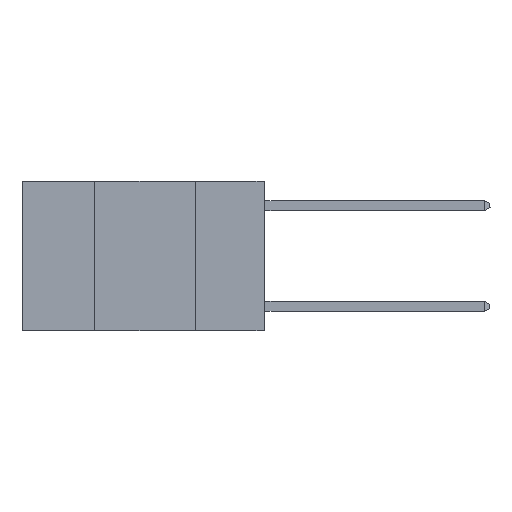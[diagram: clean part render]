
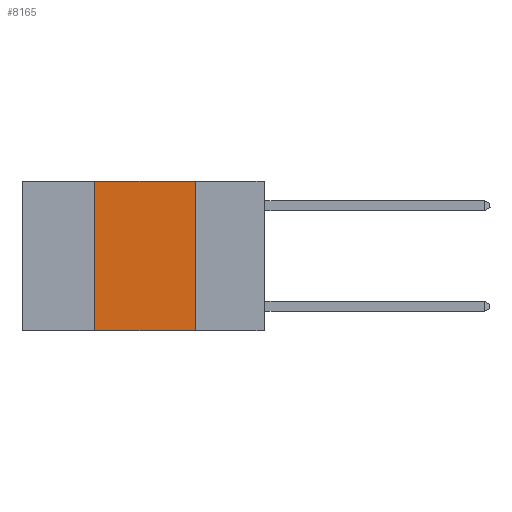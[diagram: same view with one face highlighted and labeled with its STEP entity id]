
A CAD part, left-side view. The second image highlights one B-rep face of the part: STEP entity #8165.
In plain terms, the highlighted planar face has unit normal (-1, 0, 0).
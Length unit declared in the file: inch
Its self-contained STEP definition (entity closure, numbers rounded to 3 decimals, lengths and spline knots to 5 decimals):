
#503 = VECTOR ( 'NONE', #14756, 39.37008 ) ;
#889 = EDGE_CURVE ( 'NONE', #12128, #11529, #6515, .T. ) ;
#1473 = DIRECTION ( 'NONE',  ( 1., 0., 0. ) ) ;
#2591 = LINE ( 'NONE', #10901, #12877 ) ;
#3514 = LINE ( 'NONE', #3732, #9377 ) ;
#3732 = CARTESIAN_POINT ( 'NONE',  ( 0., 0.6, -0.37 ) ) ;
#4148 = CARTESIAN_POINT ( 'NONE',  ( 0., 0.6, 0. ) ) ;
#4166 = DIRECTION ( 'NONE',  ( 0., 0., 1. ) ) ;
#4298 = CARTESIAN_POINT ( 'NONE',  ( 0., 0.17, -0.37 ) ) ;
#5715 = CARTESIAN_POINT ( 'NONE',  ( 0., 0.42, 0. ) ) ;
#6105 = VECTOR ( 'NONE', #14908, 39.37008 ) ;
#6139 = AXIS2_PLACEMENT_3D ( 'NONE', #14839, #1473, #10809 ) ;
#6515 = LINE ( 'NONE', #4148, #6105 ) ;
#6765 = PLANE ( 'NONE',  #6139 ) ;
#6842 = VERTEX_POINT ( 'NONE', #4298 ) ;
#7794 = FACE_OUTER_BOUND ( 'NONE', #10103, .T. ) ;
#8024 = CARTESIAN_POINT ( 'NONE',  ( 0., 0.17, 0. ) ) ;
#8165 = ADVANCED_FACE ( 'NONE', ( #7794 ), #6765, .F. ) ;
#8850 = EDGE_CURVE ( 'NONE', #11529, #6842, #14737, .T. ) ;
#9377 = VECTOR ( 'NONE', #14471, 39.37008 ) ;
#10103 = EDGE_LOOP ( 'NONE', ( #13173, #13599, #10405, #10841 ) ) ;
#10405 = ORIENTED_EDGE ( 'NONE', *, *, #16078, .F. ) ;
#10809 = DIRECTION ( 'NONE',  ( 0., 0., -1. ) ) ;
#10841 = ORIENTED_EDGE ( 'NONE', *, *, #11829, .T. ) ;
#10901 = CARTESIAN_POINT ( 'NONE',  ( 0., 0.42, 0. ) ) ;
#11400 = CARTESIAN_POINT ( 'NONE',  ( 0., 0.42, -0.37 ) ) ;
#11529 = VERTEX_POINT ( 'NONE', #12500 ) ;
#11829 = EDGE_CURVE ( 'NONE', #16718, #6842, #3514, .T. ) ;
#12128 = VERTEX_POINT ( 'NONE', #5715 ) ;
#12500 = CARTESIAN_POINT ( 'NONE',  ( 0., 0.17, 0. ) ) ;
#12877 = VECTOR ( 'NONE', #4166, 39.37008 ) ;
#13173 = ORIENTED_EDGE ( 'NONE', *, *, #8850, .F. ) ;
#13599 = ORIENTED_EDGE ( 'NONE', *, *, #889, .F. ) ;
#14471 = DIRECTION ( 'NONE',  ( 0., -1., 0. ) ) ;
#14737 = LINE ( 'NONE', #8024, #503 ) ;
#14756 = DIRECTION ( 'NONE',  ( 0., 0., -1. ) ) ;
#14839 = CARTESIAN_POINT ( 'NONE',  ( 0., 0.6, 0. ) ) ;
#14908 = DIRECTION ( 'NONE',  ( 0., -1., 0. ) ) ;
#16078 = EDGE_CURVE ( 'NONE', #16718, #12128, #2591, .T. ) ;
#16718 = VERTEX_POINT ( 'NONE', #11400 ) ;
